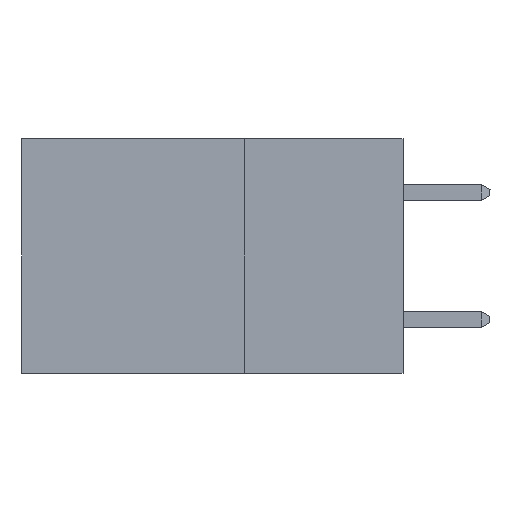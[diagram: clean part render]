
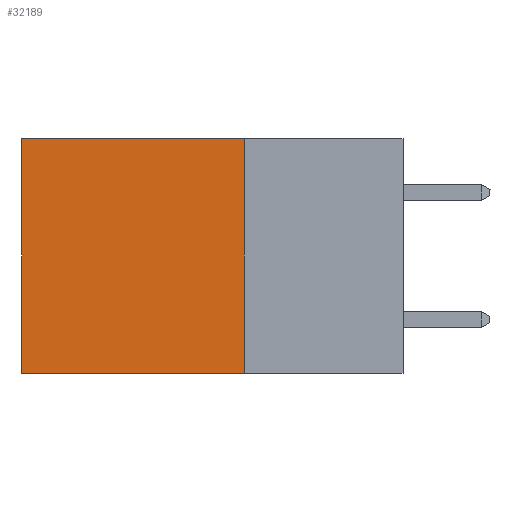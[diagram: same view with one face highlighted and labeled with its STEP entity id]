
A CAD part, left-side view. The second image highlights one B-rep face of the part: STEP entity #32189.
In plain terms, the highlighted planar face has unit normal (-1, 0, 0).
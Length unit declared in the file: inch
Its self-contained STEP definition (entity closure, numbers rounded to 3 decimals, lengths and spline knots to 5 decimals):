
#353 = EDGE_CURVE ( 'NONE', #21106, #33881, #22269, .T. ) ;
#586 = VECTOR ( 'NONE', #12228, 39.37008 ) ;
#624 = ORIENTED_EDGE ( 'NONE', *, *, #38366, .T. ) ;
#690 = CARTESIAN_POINT ( 'NONE',  ( 0.2875, 0.6, 0. ) ) ;
#4042 = PLANE ( 'NONE',  #32625 ) ;
#6969 = DIRECTION ( 'NONE',  ( 0., 1., 0. ) ) ;
#7457 = CARTESIAN_POINT ( 'NONE',  ( 0.2875, 0.25, 0. ) ) ;
#7971 = VECTOR ( 'NONE', #14415, 39.37008 ) ;
#9630 = LINE ( 'NONE', #36033, #586 ) ;
#10395 = CARTESIAN_POINT ( 'NONE',  ( 0.2875, 0.25, 0. ) ) ;
#10725 = LINE ( 'NONE', #30824, #18695 ) ;
#12228 = DIRECTION ( 'NONE',  ( 0., 1., 0. ) ) ;
#13057 = FACE_OUTER_BOUND ( 'NONE', #38650, .T. ) ;
#13615 = EDGE_CURVE ( 'NONE', #33881, #27854, #10725, .T. ) ;
#13858 = DIRECTION ( 'NONE',  ( 0., 0., -1. ) ) ;
#14312 = EDGE_CURVE ( 'NONE', #32052, #27854, #17060, .T. ) ;
#14415 = DIRECTION ( 'NONE',  ( 0., 0., -1. ) ) ;
#15689 = CARTESIAN_POINT ( 'NONE',  ( 0.2875, 0.25, -0.37 ) ) ;
#17060 = LINE ( 'NONE', #690, #7971 ) ;
#17741 = DIRECTION ( 'NONE',  ( 1., 0., 0. ) ) ;
#18695 = VECTOR ( 'NONE', #6969, 39.37008 ) ;
#20319 = ORIENTED_EDGE ( 'NONE', *, *, #13615, .F. ) ;
#21106 = VERTEX_POINT ( 'NONE', #22858 ) ;
#22269 = LINE ( 'NONE', #10395, #30253 ) ;
#22858 = CARTESIAN_POINT ( 'NONE',  ( 0.2875, 0.25, 0. ) ) ;
#23015 = ORIENTED_EDGE ( 'NONE', *, *, #14312, .T. ) ;
#23924 = CARTESIAN_POINT ( 'NONE',  ( 0.2875, 0.6, 0. ) ) ;
#27854 = VERTEX_POINT ( 'NONE', #35927 ) ;
#30253 = VECTOR ( 'NONE', #13858, 39.37008 ) ;
#30824 = CARTESIAN_POINT ( 'NONE',  ( 0.2875, 0.25, -0.37 ) ) ;
#32052 = VERTEX_POINT ( 'NONE', #23924 ) ;
#32189 = ADVANCED_FACE ( 'NONE', ( #13057 ), #4042, .F. ) ;
#32625 = AXIS2_PLACEMENT_3D ( 'NONE', #7457, #17741, #41460 ) ;
#33881 = VERTEX_POINT ( 'NONE', #15689 ) ;
#35927 = CARTESIAN_POINT ( 'NONE',  ( 0.2875, 0.6, -0.37 ) ) ;
#36033 = CARTESIAN_POINT ( 'NONE',  ( 0.2875, 0.25, 0. ) ) ;
#38143 = ORIENTED_EDGE ( 'NONE', *, *, #353, .F. ) ;
#38366 = EDGE_CURVE ( 'NONE', #21106, #32052, #9630, .T. ) ;
#38650 = EDGE_LOOP ( 'NONE', ( #23015, #20319, #38143, #624 ) ) ;
#41460 = DIRECTION ( 'NONE',  ( 0., 0., -1. ) ) ;
